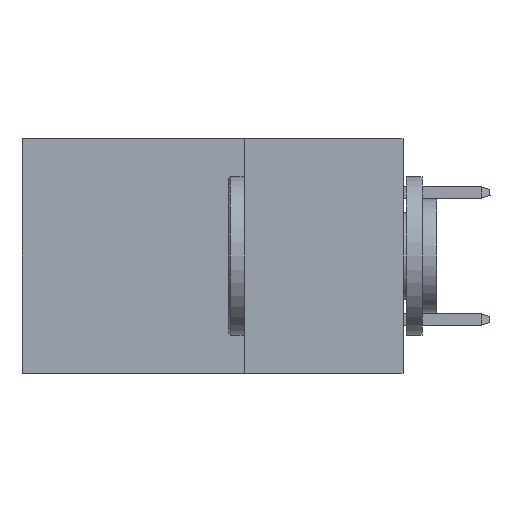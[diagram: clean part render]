
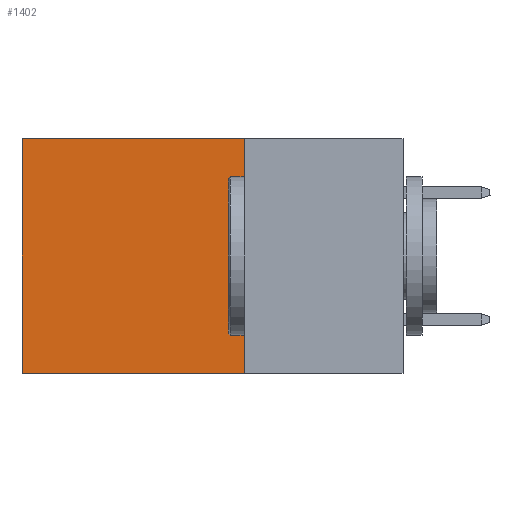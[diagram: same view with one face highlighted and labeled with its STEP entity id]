
A CAD part, left-side view. The second image highlights one B-rep face of the part: STEP entity #1402.
In plain terms, the highlighted planar face has unit normal (-1, 0, 0).
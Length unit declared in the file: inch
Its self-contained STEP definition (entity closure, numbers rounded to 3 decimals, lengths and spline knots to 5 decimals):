
#561 = LINE ( 'NONE', #39436, #10916 ) ;
#655 = ORIENTED_EDGE ( 'NONE', *, *, #27508, .F. ) ;
#1402 = ADVANCED_FACE ( 'NONE', ( #38800 ), #9972, .F. ) ;
#1529 = VERTEX_POINT ( 'NONE', #28385 ) ;
#1798 = VERTEX_POINT ( 'NONE', #40561 ) ;
#2718 = ORIENTED_EDGE ( 'NONE', *, *, #4323, .T. ) ;
#4323 = EDGE_CURVE ( 'NONE', #1529, #16619, #34684, .T. ) ;
#6815 = DIRECTION ( 'NONE',  ( 1., 0., 0. ) ) ;
#9456 = DIRECTION ( 'NONE',  ( 0., 0., -1. ) ) ;
#9592 = VECTOR ( 'NONE', #15370, 39.37008 ) ;
#9972 = PLANE ( 'NONE',  #35976 ) ;
#10916 = VECTOR ( 'NONE', #17555, 39.37008 ) ;
#12627 = LINE ( 'NONE', #21287, #9592 ) ;
#13242 = VECTOR ( 'NONE', #36842, 39.37008 ) ;
#13546 = ORIENTED_EDGE ( 'NONE', *, *, #14745, .T. ) ;
#13912 = CARTESIAN_POINT ( 'NONE',  ( 0.2875, 0.25, 0. ) ) ;
#14745 = EDGE_CURVE ( 'NONE', #16619, #28874, #32787, .T. ) ;
#15370 = DIRECTION ( 'NONE',  ( 0., 1., 0. ) ) ;
#16619 = VERTEX_POINT ( 'NONE', #20756 ) ;
#16795 = CARTESIAN_POINT ( 'NONE',  ( 0.2875, 0.6, 0. ) ) ;
#17555 = DIRECTION ( 'NONE',  ( 0., 0., -1. ) ) ;
#17981 = CARTESIAN_POINT ( 'NONE',  ( 0.2875, 0.6, -0.37 ) ) ;
#19656 = CARTESIAN_POINT ( 'NONE',  ( 0.2875, 0.25, 0. ) ) ;
#20756 = CARTESIAN_POINT ( 'NONE',  ( 0.2875, 0.6, 0. ) ) ;
#21287 = CARTESIAN_POINT ( 'NONE',  ( 0.2875, 0.25, -0.37 ) ) ;
#22694 = ORIENTED_EDGE ( 'NONE', *, *, #23867, .F. ) ;
#23867 = EDGE_CURVE ( 'NONE', #1529, #1798, #561, .T. ) ;
#26675 = DIRECTION ( 'NONE',  ( 0., 0., -1. ) ) ;
#27508 = EDGE_CURVE ( 'NONE', #1798, #28874, #12627, .T. ) ;
#28307 = EDGE_LOOP ( 'NONE', ( #13546, #655, #22694, #2718 ) ) ;
#28385 = CARTESIAN_POINT ( 'NONE',  ( 0.2875, 0.25, 0. ) ) ;
#28874 = VERTEX_POINT ( 'NONE', #17981 ) ;
#32787 = LINE ( 'NONE', #16795, #40103 ) ;
#34684 = LINE ( 'NONE', #13912, #13242 ) ;
#35976 = AXIS2_PLACEMENT_3D ( 'NONE', #19656, #6815, #9456 ) ;
#36842 = DIRECTION ( 'NONE',  ( 0., 1., 0. ) ) ;
#38800 = FACE_OUTER_BOUND ( 'NONE', #28307, .T. ) ;
#39436 = CARTESIAN_POINT ( 'NONE',  ( 0.2875, 0.25, 0. ) ) ;
#40103 = VECTOR ( 'NONE', #26675, 39.37008 ) ;
#40561 = CARTESIAN_POINT ( 'NONE',  ( 0.2875, 0.25, -0.37 ) ) ;
